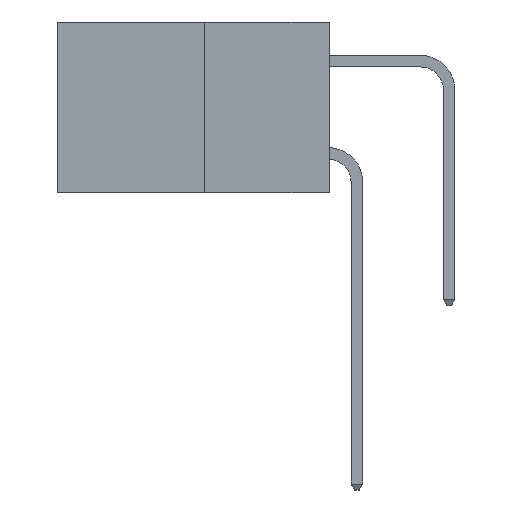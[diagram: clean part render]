
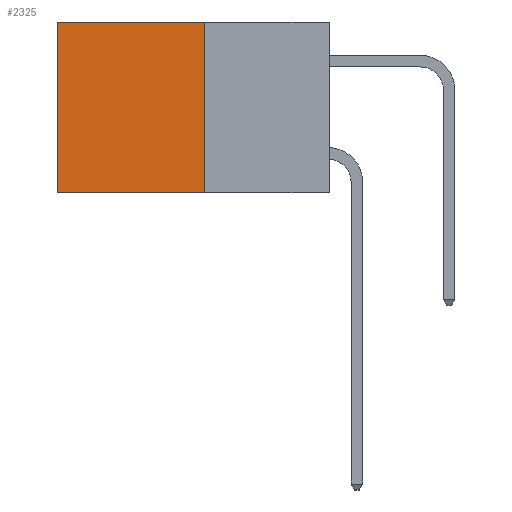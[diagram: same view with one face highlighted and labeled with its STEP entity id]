
A CAD part, left-side view. The second image highlights one B-rep face of the part: STEP entity #2325.
In plain terms, the highlighted planar face has unit normal (-1, 0, 0).
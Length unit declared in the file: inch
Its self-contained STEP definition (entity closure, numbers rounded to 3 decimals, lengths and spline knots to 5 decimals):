
#21 = ORIENTED_EDGE ( 'NONE', *, *, #10551, .T. ) ;
#66 = DIRECTION ( 'NONE',  ( 0., 0., -1. ) ) ;
#127 = PLANE ( 'NONE',  #9495 ) ;
#131 = VERTEX_POINT ( 'NONE', #11715 ) ;
#137 = EDGE_CURVE ( 'NONE', #2759, #8562, #6850, .T. ) ;
#630 = EDGE_CURVE ( 'NONE', #6435, #2759, #4633, .T. ) ;
#1257 = CARTESIAN_POINT ( 'NONE',  ( 0.277, 0.27, -0.37 ) ) ;
#1294 = CARTESIAN_POINT ( 'NONE',  ( 0.277, 0.27, -0.37 ) ) ;
#1752 = ORIENTED_EDGE ( 'NONE', *, *, #137, .F. ) ;
#2001 = VECTOR ( 'NONE', #10025, 39.37008 ) ;
#2325 = ADVANCED_FACE ( 'NONE', ( #3252 ), #127, .F. ) ;
#2329 = LINE ( 'NONE', #9142, #2001 ) ;
#2722 = DIRECTION ( 'NONE',  ( 0., 0., -1. ) ) ;
#2759 = VERTEX_POINT ( 'NONE', #1257 ) ;
#3124 = ORIENTED_EDGE ( 'NONE', *, *, #11647, .T. ) ;
#3205 = ORIENTED_EDGE ( 'NONE', *, *, #630, .F. ) ;
#3252 = FACE_OUTER_BOUND ( 'NONE', #5371, .T. ) ;
#3762 = VECTOR ( 'NONE', #66, 39.37008 ) ;
#4633 = LINE ( 'NONE', #1294, #3762 ) ;
#5001 = CARTESIAN_POINT ( 'NONE',  ( 0.277, 0.27, 0. ) ) ;
#5200 = CARTESIAN_POINT ( 'NONE',  ( 0.277, 0.59, -0.37 ) ) ;
#5371 = EDGE_LOOP ( 'NONE', ( #21, #1752, #3205, #3124 ) ) ;
#5945 = DIRECTION ( 'NONE',  ( 1., 0., 0. ) ) ;
#6435 = VERTEX_POINT ( 'NONE', #5001 ) ;
#6850 = LINE ( 'NONE', #11953, #11590 ) ;
#8562 = VERTEX_POINT ( 'NONE', #5200 ) ;
#8847 = CARTESIAN_POINT ( 'NONE',  ( 0.277, 0.59, -0.37 ) ) ;
#9142 = CARTESIAN_POINT ( 'NONE',  ( 0.277, 0.27, 0. ) ) ;
#9285 = CARTESIAN_POINT ( 'NONE',  ( 0.277, 0.27, -0.37 ) ) ;
#9495 = AXIS2_PLACEMENT_3D ( 'NONE', #9285, #5945, #2722 ) ;
#10025 = DIRECTION ( 'NONE',  ( 0., 1., 0. ) ) ;
#10551 = EDGE_CURVE ( 'NONE', #131, #8562, #11552, .T. ) ;
#11291 = VECTOR ( 'NONE', #11471, 39.37008 ) ;
#11471 = DIRECTION ( 'NONE',  ( 0., 0., -1. ) ) ;
#11552 = LINE ( 'NONE', #8847, #11291 ) ;
#11590 = VECTOR ( 'NONE', #11750, 39.37008 ) ;
#11647 = EDGE_CURVE ( 'NONE', #6435, #131, #2329, .T. ) ;
#11715 = CARTESIAN_POINT ( 'NONE',  ( 0.277, 0.59, 0. ) ) ;
#11750 = DIRECTION ( 'NONE',  ( 0., 1., 0. ) ) ;
#11953 = CARTESIAN_POINT ( 'NONE',  ( 0.277, 0.27, -0.37 ) ) ;
